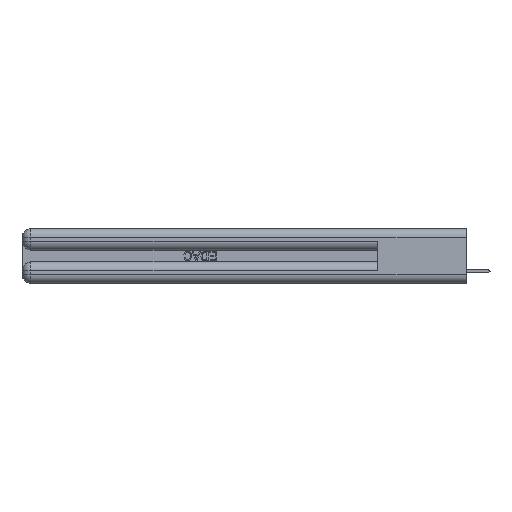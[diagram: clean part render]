
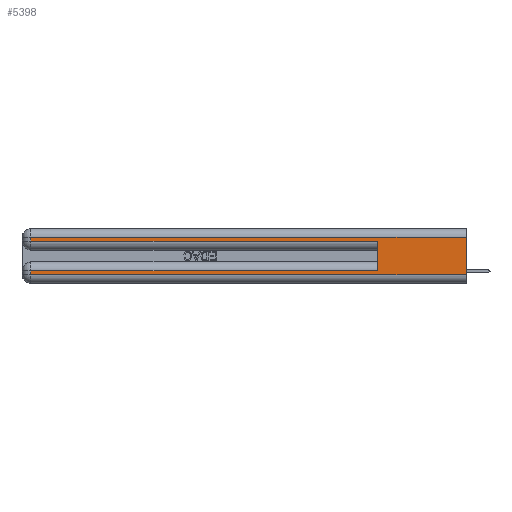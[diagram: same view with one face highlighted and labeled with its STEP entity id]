
A CAD part, left-side view. The second image highlights one B-rep face of the part: STEP entity #5398.
In plain terms, the highlighted planar face has unit normal (-1, 0, 0).
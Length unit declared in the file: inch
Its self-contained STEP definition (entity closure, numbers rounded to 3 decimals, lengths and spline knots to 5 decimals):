
#43 = ORIENTED_EDGE ( 'NONE', *, *, #51136, .T. ) ;
#267 = EDGE_CURVE ( 'NONE', #24597, #36883, #25621, .T. ) ;
#316 = VECTOR ( 'NONE', #44236, 39.37008 ) ;
#1064 = VERTEX_POINT ( 'NONE', #9563 ) ;
#1800 = VERTEX_POINT ( 'NONE', #51721 ) ;
#2196 = CARTESIAN_POINT ( 'NONE',  ( 0., 0., 0.37 ) ) ;
#2452 = DIRECTION ( 'NONE',  ( 0., 0., -1. ) ) ;
#2795 = DIRECTION ( 'NONE',  ( 0., 0., 1. ) ) ;
#3643 = LINE ( 'NONE', #42019, #21674 ) ;
#3685 = CARTESIAN_POINT ( 'NONE',  ( 0., 2.94, 0.31 ) ) ;
#4872 = EDGE_CURVE ( 'NONE', #10898, #48828, #3643, .T. ) ;
#5398 = ADVANCED_FACE ( 'NONE', ( #27887 ), #49621, .F. ) ;
#6096 = ORIENTED_EDGE ( 'NONE', *, *, #25678, .T. ) ;
#6307 = DIRECTION ( 'NONE',  ( 0., 0., -1. ) ) ;
#7334 = DIRECTION ( 'NONE',  ( 0., -1., 0. ) ) ;
#9367 = VERTEX_POINT ( 'NONE', #36419 ) ;
#9563 = CARTESIAN_POINT ( 'NONE',  ( 0., 0., 0.31 ) ) ;
#9610 = EDGE_CURVE ( 'NONE', #1064, #9367, #24998, .T. ) ;
#10157 = DIRECTION ( 'NONE',  ( 1., 0., 0. ) ) ;
#10670 = LINE ( 'NONE', #30667, #28111 ) ;
#10898 = VERTEX_POINT ( 'NONE', #18438 ) ;
#11042 = AXIS2_PLACEMENT_3D ( 'NONE', #2196, #10157, #18156 ) ;
#11477 = CARTESIAN_POINT ( 'NONE',  ( 0., 0., 0.285 ) ) ;
#11539 = VECTOR ( 'NONE', #24268, 39.37008 ) ;
#13298 = EDGE_CURVE ( 'NONE', #1800, #23519, #10670, .T. ) ;
#14224 = CARTESIAN_POINT ( 'NONE',  ( 0., 2.94, 0.37 ) ) ;
#16057 = CARTESIAN_POINT ( 'NONE',  ( 0., 0.6, 0.285 ) ) ;
#16309 = LINE ( 'NONE', #11477, #22654 ) ;
#16872 = ORIENTED_EDGE ( 'NONE', *, *, #46474, .T. ) ;
#16960 = ORIENTED_EDGE ( 'NONE', *, *, #51718, .T. ) ;
#17715 = LINE ( 'NONE', #35878, #316 ) ;
#18156 = DIRECTION ( 'NONE',  ( 0., 0., -1. ) ) ;
#18438 = CARTESIAN_POINT ( 'NONE',  ( 0., 2.94, 0.085 ) ) ;
#18688 = VECTOR ( 'NONE', #2452, 39.37008 ) ;
#19418 = ORIENTED_EDGE ( 'NONE', *, *, #4872, .T. ) ;
#20450 = CARTESIAN_POINT ( 'NONE',  ( 0., 2.94, 0.06 ) ) ;
#20510 = EDGE_LOOP ( 'NONE', ( #48829, #16960, #41204, #16872, #40145, #6096, #19418, #43 ) ) ;
#21674 = VECTOR ( 'NONE', #6307, 39.37008 ) ;
#22202 = LINE ( 'NONE', #28404, #11539 ) ;
#22654 = VECTOR ( 'NONE', #7334, 39.37008 ) ;
#23519 = VERTEX_POINT ( 'NONE', #16057 ) ;
#24268 = DIRECTION ( 'NONE',  ( 0., 1., 0. ) ) ;
#24597 = VERTEX_POINT ( 'NONE', #3685 ) ;
#24998 = LINE ( 'NONE', #26383, #41162 ) ;
#25621 = LINE ( 'NONE', #14224, #18688 ) ;
#25678 = EDGE_CURVE ( 'NONE', #1800, #10898, #22202, .T. ) ;
#26383 = CARTESIAN_POINT ( 'NONE',  ( 0., 0., 0.37 ) ) ;
#27504 = DIRECTION ( 'NONE',  ( 0., 1., 0. ) ) ;
#27887 = FACE_OUTER_BOUND ( 'NONE', #20510, .T. ) ;
#28111 = VECTOR ( 'NONE', #2795, 39.37008 ) ;
#28404 = CARTESIAN_POINT ( 'NONE',  ( 0., 0., 0.085 ) ) ;
#30667 = CARTESIAN_POINT ( 'NONE',  ( 0., 0.6, 0.145 ) ) ;
#35878 = CARTESIAN_POINT ( 'NONE',  ( 0., 0., 0.06 ) ) ;
#36419 = CARTESIAN_POINT ( 'NONE',  ( 0., 0., 0.06 ) ) ;
#36883 = VERTEX_POINT ( 'NONE', #43194 ) ;
#38250 = LINE ( 'NONE', #47216, #42029 ) ;
#40145 = ORIENTED_EDGE ( 'NONE', *, *, #13298, .F. ) ;
#41162 = VECTOR ( 'NONE', #42415, 39.37008 ) ;
#41204 = ORIENTED_EDGE ( 'NONE', *, *, #267, .T. ) ;
#42019 = CARTESIAN_POINT ( 'NONE',  ( 0., 2.94, 0.37 ) ) ;
#42029 = VECTOR ( 'NONE', #27504, 39.37008 ) ;
#42415 = DIRECTION ( 'NONE',  ( 0., 0., -1. ) ) ;
#43194 = CARTESIAN_POINT ( 'NONE',  ( 0., 2.94, 0.285 ) ) ;
#44236 = DIRECTION ( 'NONE',  ( 0., -1., 0. ) ) ;
#46474 = EDGE_CURVE ( 'NONE', #36883, #23519, #16309, .T. ) ;
#47216 = CARTESIAN_POINT ( 'NONE',  ( 0., 0., 0.31 ) ) ;
#48828 = VERTEX_POINT ( 'NONE', #20450 ) ;
#48829 = ORIENTED_EDGE ( 'NONE', *, *, #9610, .F. ) ;
#49621 = PLANE ( 'NONE',  #11042 ) ;
#51136 = EDGE_CURVE ( 'NONE', #48828, #9367, #17715, .T. ) ;
#51718 = EDGE_CURVE ( 'NONE', #1064, #24597, #38250, .T. ) ;
#51721 = CARTESIAN_POINT ( 'NONE',  ( 0., 0.6, 0.085 ) ) ;
